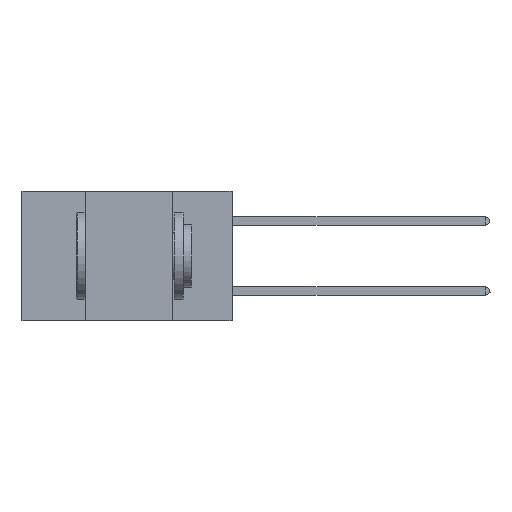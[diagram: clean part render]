
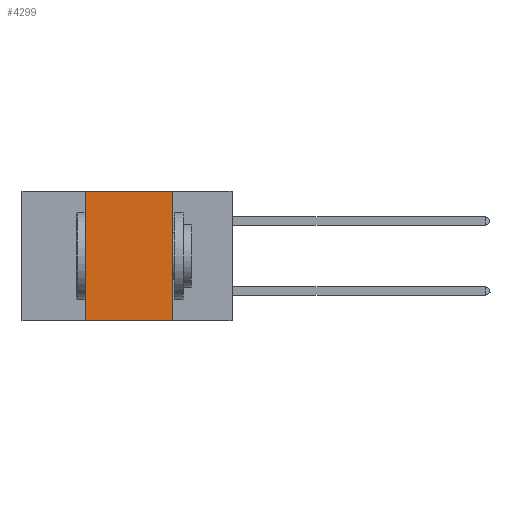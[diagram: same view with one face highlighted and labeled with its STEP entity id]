
A CAD part, left-side view. The second image highlights one B-rep face of the part: STEP entity #4299.
In plain terms, the highlighted planar face has unit normal (-1, 0, 0).
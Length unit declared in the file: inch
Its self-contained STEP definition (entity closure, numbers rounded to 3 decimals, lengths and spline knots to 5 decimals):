
#1045 = CARTESIAN_POINT ( 'NONE',  ( 0., 0.17, 0. ) ) ;
#1458 = VECTOR ( 'NONE', #4648, 39.37008 ) ;
#2301 = DIRECTION ( 'NONE',  ( 0., -1., 0. ) ) ;
#2365 = VECTOR ( 'NONE', #14051, 39.37008 ) ;
#2571 = VERTEX_POINT ( 'NONE', #41502 ) ;
#3026 = DIRECTION ( 'NONE',  ( 1., 0., 0. ) ) ;
#4299 = ADVANCED_FACE ( 'NONE', ( #37425 ), #42189, .F. ) ;
#4648 = DIRECTION ( 'NONE',  ( 0., 0., -1. ) ) ;
#4936 = VECTOR ( 'NONE', #2301, 39.37008 ) ;
#5623 = DIRECTION ( 'NONE',  ( 0., -1., 0. ) ) ;
#9213 = ORIENTED_EDGE ( 'NONE', *, *, #23947, .F. ) ;
#10419 = CARTESIAN_POINT ( 'NONE',  ( 0., 0.42, 0. ) ) ;
#11911 = LINE ( 'NONE', #10419, #2365 ) ;
#13137 = VERTEX_POINT ( 'NONE', #34167 ) ;
#13516 = VERTEX_POINT ( 'NONE', #18182 ) ;
#14051 = DIRECTION ( 'NONE',  ( 0., 0., 1. ) ) ;
#16949 = EDGE_CURVE ( 'NONE', #13137, #13516, #11911, .T. ) ;
#18182 = CARTESIAN_POINT ( 'NONE',  ( 0., 0.42, 0. ) ) ;
#18756 = EDGE_CURVE ( 'NONE', #13137, #39518, #33596, .T. ) ;
#19448 = AXIS2_PLACEMENT_3D ( 'NONE', #38677, #3026, #28227 ) ;
#20008 = ORIENTED_EDGE ( 'NONE', *, *, #16949, .F. ) ;
#23947 = EDGE_CURVE ( 'NONE', #2571, #39518, #39488, .T. ) ;
#27240 = CARTESIAN_POINT ( 'NONE',  ( 0., 0.6, 0. ) ) ;
#28227 = DIRECTION ( 'NONE',  ( 0., 0., -1. ) ) ;
#29568 = ORIENTED_EDGE ( 'NONE', *, *, #18756, .T. ) ;
#32725 = EDGE_CURVE ( 'NONE', #13516, #2571, #39659, .T. ) ;
#33596 = LINE ( 'NONE', #45118, #4936 ) ;
#34167 = CARTESIAN_POINT ( 'NONE',  ( 0., 0.42, -0.37 ) ) ;
#35976 = EDGE_LOOP ( 'NONE', ( #9213, #43783, #20008, #29568 ) ) ;
#37425 = FACE_OUTER_BOUND ( 'NONE', #35976, .T. ) ;
#38677 = CARTESIAN_POINT ( 'NONE',  ( 0., 0.6, 0. ) ) ;
#38918 = CARTESIAN_POINT ( 'NONE',  ( 0., 0.17, -0.37 ) ) ;
#39488 = LINE ( 'NONE', #1045, #1458 ) ;
#39518 = VERTEX_POINT ( 'NONE', #38918 ) ;
#39659 = LINE ( 'NONE', #27240, #40757 ) ;
#40757 = VECTOR ( 'NONE', #5623, 39.37008 ) ;
#41502 = CARTESIAN_POINT ( 'NONE',  ( 0., 0.17, 0. ) ) ;
#42189 = PLANE ( 'NONE',  #19448 ) ;
#43783 = ORIENTED_EDGE ( 'NONE', *, *, #32725, .F. ) ;
#45118 = CARTESIAN_POINT ( 'NONE',  ( 0., 0.6, -0.37 ) ) ;
